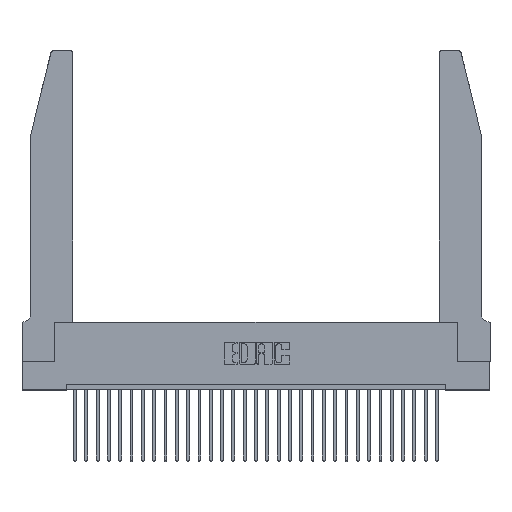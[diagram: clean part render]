
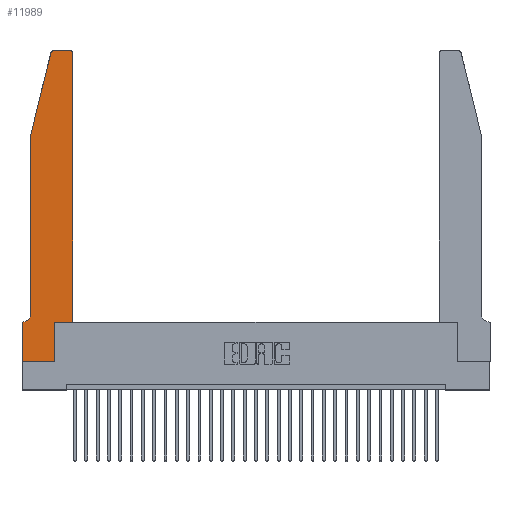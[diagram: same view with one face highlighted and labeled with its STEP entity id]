
A CAD part, top view. The second image highlights one B-rep face of the part: STEP entity #11989.
In plain terms, the highlighted planar face has unit normal (0, 0, 1).
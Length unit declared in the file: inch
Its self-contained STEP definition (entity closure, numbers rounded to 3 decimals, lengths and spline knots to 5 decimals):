
#218 = EDGE_CURVE ( 'NONE', #19779, #15092, #14906, .T. ) ;
#476 = CARTESIAN_POINT ( 'NONE',  ( 0.4205, 2.75, 0.37 ) ) ;
#949 = CARTESIAN_POINT ( 'NONE',  ( 0.4505, 0.35, 0.37 ) ) ;
#1183 = CARTESIAN_POINT ( 'NONE',  ( 0., 0., 0.37 ) ) ;
#1768 = AXIS2_PLACEMENT_3D ( 'NONE', #12681, #15383, #3307 ) ;
#2342 = CARTESIAN_POINT ( 'NONE',  ( 0., 0.35, 0.37 ) ) ;
#3210 = EDGE_CURVE ( 'NONE', #25718, #26709, #26930, .T. ) ;
#3307 = DIRECTION ( 'NONE',  ( 1., 0., 0. ) ) ;
#3711 = CARTESIAN_POINT ( 'NONE',  ( 0.2865, 0.35, 0.37 ) ) ;
#3830 = ORIENTED_EDGE ( 'NONE', *, *, #7568, .T. ) ;
#4019 = LINE ( 'NONE', #9345, #27831 ) ;
#4316 = EDGE_CURVE ( 'NONE', #13001, #15365, #11645, .T. ) ;
#4711 = DIRECTION ( 'NONE',  ( 0., 0., 1. ) ) ;
#4841 = VERTEX_POINT ( 'NONE', #7125 ) ;
#4989 = ORIENTED_EDGE ( 'NONE', *, *, #4316, .T. ) ;
#5113 = CARTESIAN_POINT ( 'NONE',  ( 0., 0., 0.37 ) ) ;
#5754 = DIRECTION ( 'NONE',  ( -1., 0., 0. ) ) ;
#6128 = CIRCLE ( 'NONE', #10068, 0.03 ) ;
#6306 = LINE ( 'NONE', #13550, #25293 ) ;
#6349 = EDGE_LOOP ( 'NONE', ( #22411, #29516, #16725, #3830, #4989, #22924, #14541, #18018, #22749, #28560, #9829, #20620 ) ) ;
#6476 = DIRECTION ( 'NONE',  ( -1., 0., 0. ) ) ;
#7036 = VERTEX_POINT ( 'NONE', #7071 ) ;
#7071 = CARTESIAN_POINT ( 'NONE',  ( 0.284, 2.75, 0.37 ) ) ;
#7125 = CARTESIAN_POINT ( 'NONE',  ( 0., 0.35, 0.37 ) ) ;
#7171 = CARTESIAN_POINT ( 'NONE',  ( 0.2865, 0., 0.37 ) ) ;
#7272 = DIRECTION ( 'NONE',  ( 1., 0., 0. ) ) ;
#7568 = EDGE_CURVE ( 'NONE', #26709, #13001, #18074, .T. ) ;
#7747 = DIRECTION ( 'NONE',  ( 1., 0., 0. ) ) ;
#7937 = DIRECTION ( 'NONE',  ( 1., 0., 0. ) ) ;
#8180 = CARTESIAN_POINT ( 'NONE',  ( 0.0755, 0.42, 0.37 ) ) ;
#8478 = VERTEX_POINT ( 'NONE', #7171 ) ;
#9235 = VECTOR ( 'NONE', #7937, 39.37008 ) ;
#9250 = AXIS2_PLACEMENT_3D ( 'NONE', #2342, #4711, #23721 ) ;
#9345 = CARTESIAN_POINT ( 'NONE',  ( 0., 0., 0.37 ) ) ;
#9796 = CARTESIAN_POINT ( 'NONE',  ( 0.0055, 0.35, 0.37 ) ) ;
#9829 = ORIENTED_EDGE ( 'NONE', *, *, #29402, .T. ) ;
#10068 = AXIS2_PLACEMENT_3D ( 'NONE', #21516, #26400, #7272 ) ;
#10666 = CARTESIAN_POINT ( 'NONE',  ( 0.4505, 0.35, 0.37 ) ) ;
#11059 = LINE ( 'NONE', #10666, #11813 ) ;
#11157 = VERTEX_POINT ( 'NONE', #12345 ) ;
#11645 = CIRCLE ( 'NONE', #23744, 0.07 ) ;
#11813 = VECTOR ( 'NONE', #7747, 39.37008 ) ;
#11989 = ADVANCED_FACE ( 'NONE', ( #19556 ), #16584, .T. ) ;
#12120 = DIRECTION ( 'NONE',  ( 0., 0., -1. ) ) ;
#12345 = CARTESIAN_POINT ( 'NONE',  ( 0.2865, 0.35, 0.37 ) ) ;
#12681 = CARTESIAN_POINT ( 'NONE',  ( 0.4205, 2.72, 0.37 ) ) ;
#12698 = LINE ( 'NONE', #3711, #14205 ) ;
#13001 = VERTEX_POINT ( 'NONE', #8180 ) ;
#13549 = DIRECTION ( 'NONE',  ( -0.239, -0.971, 0. ) ) ;
#13550 = CARTESIAN_POINT ( 'NONE',  ( 0.0755, 0.35, 0.37 ) ) ;
#14205 = VECTOR ( 'NONE', #20160, 39.37008 ) ;
#14541 = ORIENTED_EDGE ( 'NONE', *, *, #27698, .T. ) ;
#14906 = CIRCLE ( 'NONE', #1768, 0.03 ) ;
#15081 = LINE ( 'NONE', #949, #29984 ) ;
#15092 = VERTEX_POINT ( 'NONE', #476 ) ;
#15113 = CARTESIAN_POINT ( 'NONE',  ( 0.2605, 2.75, 0.37 ) ) ;
#15365 = VERTEX_POINT ( 'NONE', #9796 ) ;
#15383 = DIRECTION ( 'NONE',  ( 0., 0., 1. ) ) ;
#16231 = DIRECTION ( 'NONE',  ( 0., -1., 0. ) ) ;
#16584 = PLANE ( 'NONE',  #9250 ) ;
#16620 = DIRECTION ( 'NONE',  ( -1., 0., 0. ) ) ;
#16725 = ORIENTED_EDGE ( 'NONE', *, *, #3210, .T. ) ;
#17585 = DIRECTION ( 'NONE',  ( 0., 1., 0. ) ) ;
#17736 = CARTESIAN_POINT ( 'NONE',  ( 0.0055, 0.42, 0.37 ) ) ;
#18018 = ORIENTED_EDGE ( 'NONE', *, *, #23606, .T. ) ;
#18074 = LINE ( 'NONE', #21258, #29718 ) ;
#18129 = EDGE_CURVE ( 'NONE', #8478, #11157, #12698, .T. ) ;
#19213 = VERTEX_POINT ( 'NONE', #5113 ) ;
#19478 = CARTESIAN_POINT ( 'NONE',  ( 0.0755, 2., 0.37 ) ) ;
#19556 = FACE_OUTER_BOUND ( 'NONE', #6349, .T. ) ;
#19779 = VERTEX_POINT ( 'NONE', #24278 ) ;
#20160 = DIRECTION ( 'NONE',  ( 0., 1., 0. ) ) ;
#20620 = ORIENTED_EDGE ( 'NONE', *, *, #218, .T. ) ;
#21258 = CARTESIAN_POINT ( 'NONE',  ( 0.0755, 2., 0.37 ) ) ;
#21516 = CARTESIAN_POINT ( 'NONE',  ( 0.284, 2.72, 0.37 ) ) ;
#22142 = VERTEX_POINT ( 'NONE', #23307 ) ;
#22411 = ORIENTED_EDGE ( 'NONE', *, *, #27943, .T. ) ;
#22641 = EDGE_CURVE ( 'NONE', #15365, #4841, #6306, .T. ) ;
#22749 = ORIENTED_EDGE ( 'NONE', *, *, #18129, .T. ) ;
#22924 = ORIENTED_EDGE ( 'NONE', *, *, #22641, .T. ) ;
#23307 = CARTESIAN_POINT ( 'NONE',  ( 0.4505, 0.35, 0.37 ) ) ;
#23606 = EDGE_CURVE ( 'NONE', #19213, #8478, #27841, .T. ) ;
#23721 = DIRECTION ( 'NONE',  ( 1., 0., 0. ) ) ;
#23744 = AXIS2_PLACEMENT_3D ( 'NONE', #17736, #12120, #16620 ) ;
#24278 = CARTESIAN_POINT ( 'NONE',  ( 0.4505, 2.72, 0.37 ) ) ;
#24349 = VECTOR ( 'NONE', #13549, 39.37008 ) ;
#25217 = LINE ( 'NONE', #15113, #26698 ) ;
#25293 = VECTOR ( 'NONE', #6476, 39.37008 ) ;
#25591 = EDGE_CURVE ( 'NONE', #7036, #25718, #6128, .T. ) ;
#25718 = VERTEX_POINT ( 'NONE', #29315 ) ;
#26400 = DIRECTION ( 'NONE',  ( 0., 0., 1. ) ) ;
#26698 = VECTOR ( 'NONE', #5754, 39.37008 ) ;
#26709 = VERTEX_POINT ( 'NONE', #19478 ) ;
#26930 = LINE ( 'NONE', #30214, #24349 ) ;
#27698 = EDGE_CURVE ( 'NONE', #4841, #19213, #4019, .T. ) ;
#27831 = VECTOR ( 'NONE', #16231, 39.37008 ) ;
#27841 = LINE ( 'NONE', #1183, #9235 ) ;
#27943 = EDGE_CURVE ( 'NONE', #15092, #7036, #25217, .T. ) ;
#28085 = EDGE_CURVE ( 'NONE', #11157, #22142, #11059, .T. ) ;
#28434 = DIRECTION ( 'NONE',  ( 0., -1., 0. ) ) ;
#28560 = ORIENTED_EDGE ( 'NONE', *, *, #28085, .T. ) ;
#29315 = CARTESIAN_POINT ( 'NONE',  ( 0.25487, 2.72718, 0.37 ) ) ;
#29402 = EDGE_CURVE ( 'NONE', #22142, #19779, #15081, .T. ) ;
#29516 = ORIENTED_EDGE ( 'NONE', *, *, #25591, .T. ) ;
#29718 = VECTOR ( 'NONE', #28434, 39.37008 ) ;
#29984 = VECTOR ( 'NONE', #17585, 39.37008 ) ;
#30214 = CARTESIAN_POINT ( 'NONE',  ( 0.0755, 2., 0.37 ) ) ;
